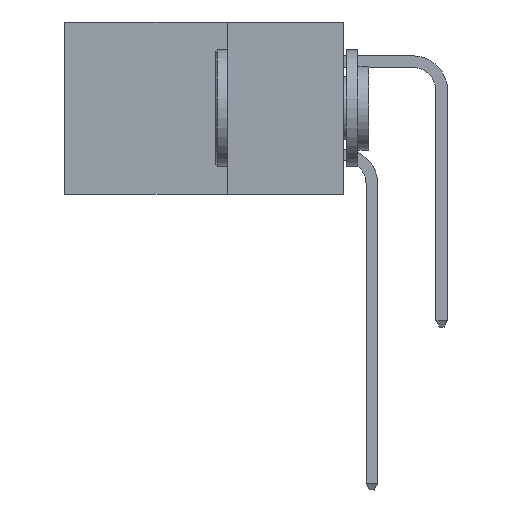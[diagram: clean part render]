
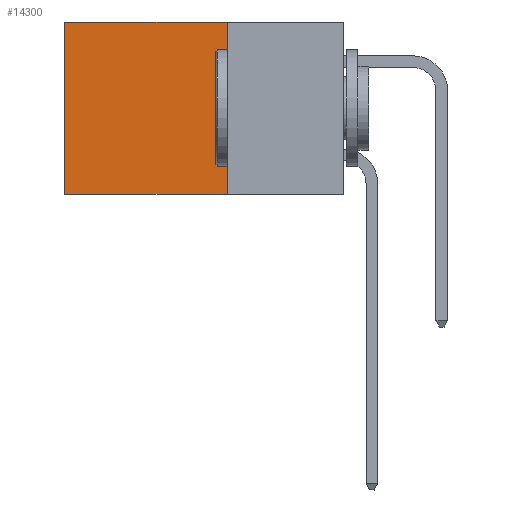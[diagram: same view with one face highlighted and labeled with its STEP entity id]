
A CAD part, left-side view. The second image highlights one B-rep face of the part: STEP entity #14300.
In plain terms, the highlighted planar face has unit normal (-1, 0, 0).
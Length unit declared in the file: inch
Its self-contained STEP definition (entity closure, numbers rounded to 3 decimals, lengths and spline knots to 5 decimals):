
#571 = ORIENTED_EDGE ( 'NONE', *, *, #15811, .T. ) ;
#1696 = VECTOR ( 'NONE', #19087, 39.37008 ) ;
#2563 = AXIS2_PLACEMENT_3D ( 'NONE', #10590, #2676, #21275 ) ;
#2676 = DIRECTION ( 'NONE',  ( 1., 0., 0. ) ) ;
#3127 = CARTESIAN_POINT ( 'NONE',  ( 0.298, 0.25, -0.37 ) ) ;
#5518 = CARTESIAN_POINT ( 'NONE',  ( 0.298, 0.6, -0.37 ) ) ;
#5548 = VERTEX_POINT ( 'NONE', #5518 ) ;
#6300 = VERTEX_POINT ( 'NONE', #26293 ) ;
#6456 = CARTESIAN_POINT ( 'NONE',  ( 0.298, 0.25, 0. ) ) ;
#7227 = ORIENTED_EDGE ( 'NONE', *, *, #23787, .T. ) ;
#8856 = DIRECTION ( 'NONE',  ( 0., 0., -1. ) ) ;
#9073 = EDGE_LOOP ( 'NONE', ( #571, #26304, #22091, #7227 ) ) ;
#9493 = EDGE_CURVE ( 'NONE', #19306, #5548, #29924, .T. ) ;
#10590 = CARTESIAN_POINT ( 'NONE',  ( 0.298, 0.25, 0. ) ) ;
#12382 = VERTEX_POINT ( 'NONE', #29125 ) ;
#14108 = LINE ( 'NONE', #6456, #14925 ) ;
#14300 = ADVANCED_FACE ( 'NONE', ( #20943 ), #18624, .F. ) ;
#14925 = VECTOR ( 'NONE', #22321, 39.37008 ) ;
#15811 = EDGE_CURVE ( 'NONE', #12382, #5548, #28228, .T. ) ;
#18624 = PLANE ( 'NONE',  #2563 ) ;
#19087 = DIRECTION ( 'NONE',  ( 0., 1., 0. ) ) ;
#19306 = VERTEX_POINT ( 'NONE', #30225 ) ;
#20943 = FACE_OUTER_BOUND ( 'NONE', #9073, .T. ) ;
#20990 = CARTESIAN_POINT ( 'NONE',  ( 0.298, 0.25, 0. ) ) ;
#21275 = DIRECTION ( 'NONE',  ( 0., 0., -1. ) ) ;
#22058 = CARTESIAN_POINT ( 'NONE',  ( 0.298, 0.6, 0. ) ) ;
#22091 = ORIENTED_EDGE ( 'NONE', *, *, #28248, .F. ) ;
#22321 = DIRECTION ( 'NONE',  ( 0., 1., 0. ) ) ;
#22767 = VECTOR ( 'NONE', #23616, 39.37008 ) ;
#23616 = DIRECTION ( 'NONE',  ( 0., 0., -1. ) ) ;
#23787 = EDGE_CURVE ( 'NONE', #6300, #12382, #14108, .T. ) ;
#26293 = CARTESIAN_POINT ( 'NONE',  ( 0.298, 0.25, 0. ) ) ;
#26304 = ORIENTED_EDGE ( 'NONE', *, *, #9493, .F. ) ;
#27413 = VECTOR ( 'NONE', #8856, 39.37008 ) ;
#28228 = LINE ( 'NONE', #22058, #27413 ) ;
#28248 = EDGE_CURVE ( 'NONE', #6300, #19306, #30651, .T. ) ;
#29125 = CARTESIAN_POINT ( 'NONE',  ( 0.298, 0.6, 0. ) ) ;
#29924 = LINE ( 'NONE', #3127, #1696 ) ;
#30225 = CARTESIAN_POINT ( 'NONE',  ( 0.298, 0.25, -0.37 ) ) ;
#30651 = LINE ( 'NONE', #20990, #22767 ) ;
